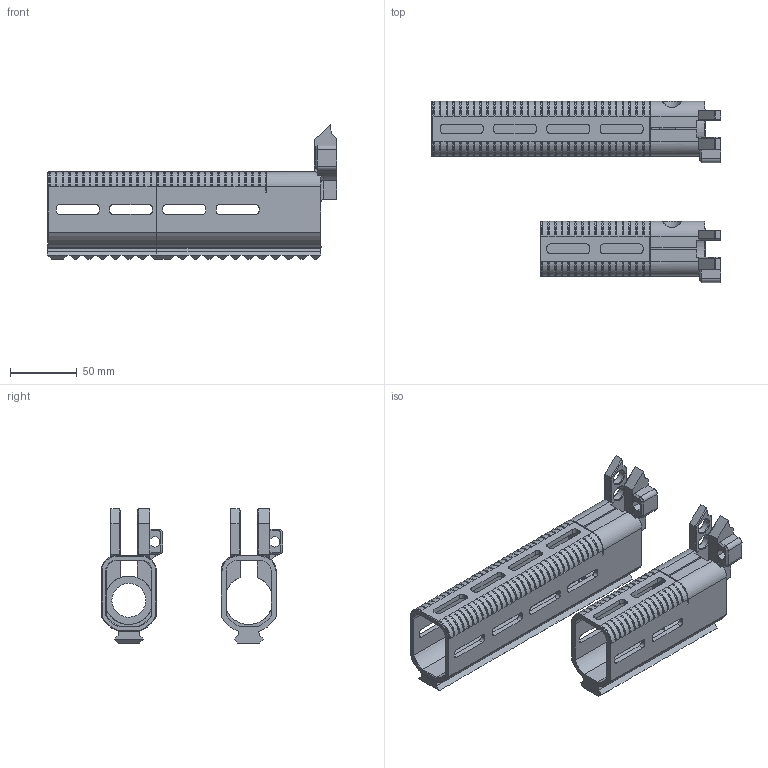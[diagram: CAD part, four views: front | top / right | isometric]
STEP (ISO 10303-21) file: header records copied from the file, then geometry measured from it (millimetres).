
FILE_DESCRIPTION(/* description */ (''),/* implementation_level */ '2;1');
FILE_NAME(/* name */ 'Tubee-22 Handguard FINAL.step',/* time_stamp */ '2021-06-23T15:50:22-04:00',/* author */ (''),/* organization */ (''),/* preprocessor_version */ 'ST-DEVELOPER v18.1',/* originating_system */ 'Autodesk Translation Framework v10.9.0.1377',/* authorisation */ '');
FILE_SCHEMA (('AUTOMOTIVE_DESIGN { 1 0 10303 214 3 1 1 }'));
Length unit declared in the file: millimetre
Products named in the file (3): Tubee-22; Thick Barrel Nut for 3d Barrel 100 thou deeper.step; handguard w rail.step
Assembly tree (2 placements, depth 2):
  Tubee-22
    Thick Barrel Nut for 3d Barrel 100 thou deeper.step
    handguard w rail.step
Bounding box: 216.9 x 135.98 x 100.84 mm (x, y, z)
Volume: 288687.8 mm3; surface area: 140651.6 mm2
Topology: 3 solids, 3 shells, 1424 faces, 3589 edges, 2177 vertices
Faces by surface type: plane 842, cylinder 405, torus 106, cone 59, bspline 12
Full cylindrical faces by diameter (mm): 9.902 x14, 11.43 x26, 12.43 x8, 14.478 x4, 25.391 x1, 30.118 x1, 30.166 x1, 32.493 x3, 35.56 x1, 36.246 x1
Entity records: 47765 total; most frequent: CARTESIAN_POINT 13454, ORIENTED_EDGE 7178, DIRECTION 7158, EDGE_CURVE 3589, AXIS2_PLACEMENT_3D 2399, LINE 2360, VECTOR 2360, VERTEX_POINT 2177
